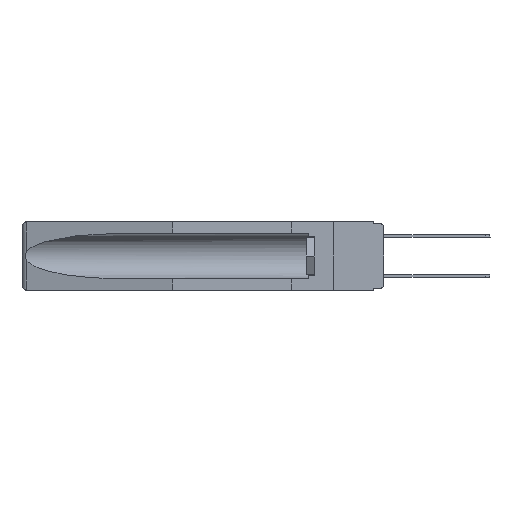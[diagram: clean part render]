
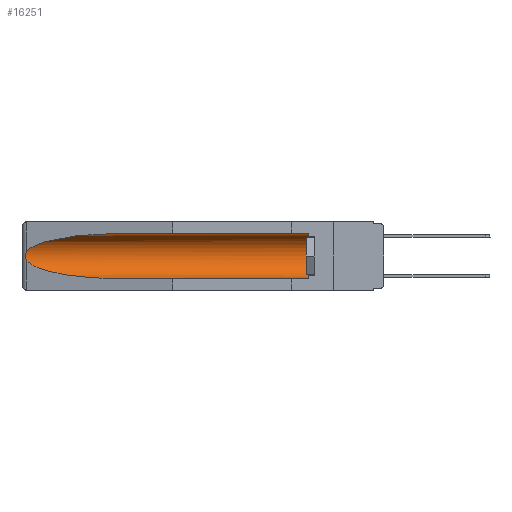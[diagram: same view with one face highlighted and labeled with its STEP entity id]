
A CAD part, left-side view. The second image highlights one B-rep face of the part: STEP entity #16251.
In plain terms, the highlighted cylindrical face has radius 2.857 mm (diameter 5.715 mm), a partial arc.
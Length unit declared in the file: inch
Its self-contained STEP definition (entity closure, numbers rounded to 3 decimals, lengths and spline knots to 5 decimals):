
#174 = CARTESIAN_POINT ( 'NONE',  ( 0.26537, 1.52718, -0.14972 ) ) ;
#376 = VERTEX_POINT ( 'NONE', #13043 ) ;
#611 = CARTESIAN_POINT ( 'NONE',  ( 0.155, 0.126, -0.284 ) ) ;
#829 = CARTESIAN_POINT ( 'NONE',  ( 0.26537, 1.52718, -0.14972 ) ) ;
#1383 = CARTESIAN_POINT ( 'NONE',  ( 0.26537, 1.52718, -0.19328 ) ) ;
#1477 = VERTEX_POINT ( 'NONE', #611 ) ;
#1489 = ORIENTED_EDGE ( 'NONE', *, *, #18286, .T. ) ;
#2211 = CARTESIAN_POINT ( 'NONE',  ( 0.21114, 1.30732, -0.059 ) ) ;
#2253 = ORIENTED_EDGE ( 'NONE', *, *, #14864, .T. ) ;
#2585 = CARTESIAN_POINT ( 'NONE',  ( 0.25451, 1.48313, -0.09465 ) ) ;
#4047 = CARTESIAN_POINT ( 'NONE',  ( 0.26537, 1.52718, -0.19328 ) ) ;
#4279 = VERTEX_POINT ( 'NONE', #4047 ) ;
#4838 = DIRECTION ( 'NONE',  ( 0., 1., 0. ) ) ;
#4964 = DIRECTION ( 'NONE',  ( 0., 0., 1. ) ) ;
#5088 = CARTESIAN_POINT ( 'NONE',  ( 0.2673, 1.5327, -0.16383 ) ) ;
#5586 = VERTEX_POINT ( 'NONE', #14208 ) ;
#5628 = DIRECTION ( 'NONE',  ( 0., 1., 0. ) ) ;
#7189 = AXIS2_PLACEMENT_3D ( 'NONE', #11586, #19279, #20908 ) ;
#7439 = EDGE_CURVE ( 'NONE', #5586, #10698, #13204, .T. ) ;
#8254 = CARTESIAN_POINT ( 'NONE',  ( 0.155, 1.07973, -0.059 ) ) ;
#8292 = CARTESIAN_POINT ( 'NONE',  ( 0.21114, 1.30732, -0.284 ) ) ;
#8793 = CARTESIAN_POINT ( 'NONE',  ( 0.26597, 1.52961, -0.15275 ) ) ;
#9266 = ORIENTED_EDGE ( 'NONE', *, *, #19553, .F. ) ;
#9450 = CARTESIAN_POINT ( 'NONE',  ( 0.155, -0.30754, -0.059 ) ) ;
#9576 = CARTESIAN_POINT ( 'NONE',  ( 0.155, -0.30754, -0.284 ) ) ;
#10698 = VERTEX_POINT ( 'NONE', #174 ) ;
#10772 = CARTESIAN_POINT ( 'NONE',  ( 0.26655, 1.53094, -0.18657 ) ) ;
#11189 = VECTOR ( 'NONE', #18985, 39.37008 ) ;
#11427 = LINE ( 'NONE', #9576, #11189 ) ;
#11586 = CARTESIAN_POINT ( 'NONE',  ( 0.155, 0.126, -0.1715 ) ) ;
#12119 =( BOUNDED_CURVE ( )  B_SPLINE_CURVE ( 3, ( #21812, #14244, #8292, #19962 ),
 .UNSPECIFIED., .F., .T. ) 
 B_SPLINE_CURVE_WITH_KNOTS ( ( 4, 4 ),
 ( 0.1948, 1.5708 ),
 .UNSPECIFIED. ) 
 CURVE ( )  GEOMETRIC_REPRESENTATION_ITEM ( )  RATIONAL_B_SPLINE_CURVE ( ( 1., 0.848, 0.848, 1. ) ) 
 REPRESENTATION_ITEM ( '' )  );
#12234 = VECTOR ( 'NONE', #5628, 39.37008 ) ;
#12617 = CARTESIAN_POINT ( 'NONE',  ( 0.2675, 1.53308, -0.16763 ) ) ;
#12692 = EDGE_CURVE ( 'NONE', #10698, #4279, #13664, .T. ) ;
#12871 = CARTESIAN_POINT ( 'NONE',  ( 0.2675, 1.53308, -0.17534 ) ) ;
#13043 = CARTESIAN_POINT ( 'NONE',  ( 0.155, 1.07973, -0.284 ) ) ;
#13204 =( BOUNDED_CURVE ( )  B_SPLINE_CURVE ( 3, ( #8254, #2211, #2585, #829 ),
 .UNSPECIFIED., .F., .T. ) 
 B_SPLINE_CURVE_WITH_KNOTS ( ( 4, 4 ),
 ( 4.71239, 6.08839 ),
 .UNSPECIFIED. ) 
 CURVE ( )  GEOMETRIC_REPRESENTATION_ITEM ( )  RATIONAL_B_SPLINE_CURVE ( ( 1., 0.848, 0.848, 1. ) ) 
 REPRESENTATION_ITEM ( '' )  );
#13664 = B_SPLINE_CURVE_WITH_KNOTS ( 'NONE', 3,
 ( #14732, #8793, #22059, #5088, #12617, #12871, #20463, #10772, #18327, #1383 ),
 .UNSPECIFIED., .F., .F.,
 ( 4, 2, 2, 2, 4 ),
 ( 0., 0.00029, 0.00058, 0.00087, 0.00117 ),
 .UNSPECIFIED. ) ;
#14208 = CARTESIAN_POINT ( 'NONE',  ( 0.155, 1.07973, -0.059 ) ) ;
#14244 = CARTESIAN_POINT ( 'NONE',  ( 0.25451, 1.48313, -0.24835 ) ) ;
#14732 = CARTESIAN_POINT ( 'NONE',  ( 0.26537, 1.52718, -0.14972 ) ) ;
#14864 = EDGE_CURVE ( 'NONE', #4279, #376, #12119, .T. ) ;
#15837 = EDGE_LOOP ( 'NONE', ( #22473, #18116, #2253, #9266, #1489, #20526 ) ) ;
#16251 = ADVANCED_FACE ( 'NONE', ( #21814 ), #16352, .F. ) ;
#16352 = CYLINDRICAL_SURFACE ( 'NONE', #18186, 0.1125 ) ;
#18086 = CARTESIAN_POINT ( 'NONE',  ( 0.155, -0.30754, -0.1715 ) ) ;
#18116 = ORIENTED_EDGE ( 'NONE', *, *, #12692, .T. ) ;
#18186 = AXIS2_PLACEMENT_3D ( 'NONE', #18086, #4838, #4964 ) ;
#18286 = EDGE_CURVE ( 'NONE', #1477, #19677, #22225, .T. ) ;
#18327 = CARTESIAN_POINT ( 'NONE',  ( 0.26597, 1.5296, -0.19026 ) ) ;
#18624 = LINE ( 'NONE', #9450, #12234 ) ;
#18985 = DIRECTION ( 'NONE',  ( 0., 1., 0. ) ) ;
#19279 = DIRECTION ( 'NONE',  ( 0., -1., 0. ) ) ;
#19499 = CARTESIAN_POINT ( 'NONE',  ( 0.155, 0.126, -0.059 ) ) ;
#19553 = EDGE_CURVE ( 'NONE', #1477, #376, #11427, .T. ) ;
#19677 = VERTEX_POINT ( 'NONE', #19499 ) ;
#19962 = CARTESIAN_POINT ( 'NONE',  ( 0.155, 1.07973, -0.284 ) ) ;
#20463 = CARTESIAN_POINT ( 'NONE',  ( 0.2673, 1.53269, -0.17917 ) ) ;
#20526 = ORIENTED_EDGE ( 'NONE', *, *, #23072, .T. ) ;
#20908 = DIRECTION ( 'NONE',  ( 0., 0., 1. ) ) ;
#21812 = CARTESIAN_POINT ( 'NONE',  ( 0.26537, 1.52718, -0.19328 ) ) ;
#21814 = FACE_OUTER_BOUND ( 'NONE', #15837, .T. ) ;
#22059 = CARTESIAN_POINT ( 'NONE',  ( 0.26654, 1.53092, -0.15636 ) ) ;
#22225 = CIRCLE ( 'NONE', #7189, 0.1125 ) ;
#22473 = ORIENTED_EDGE ( 'NONE', *, *, #7439, .T. ) ;
#23072 = EDGE_CURVE ( 'NONE', #19677, #5586, #18624, .T. ) ;
